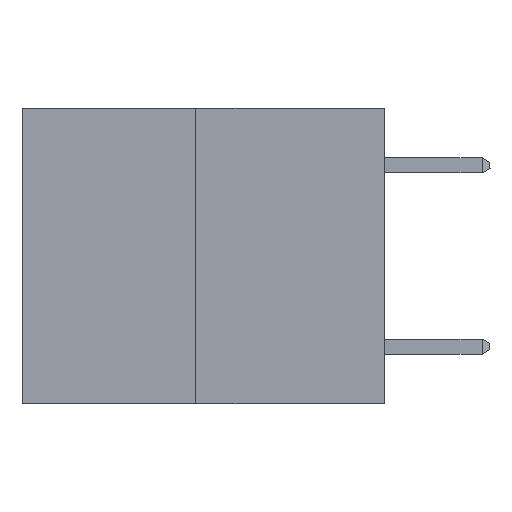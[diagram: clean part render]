
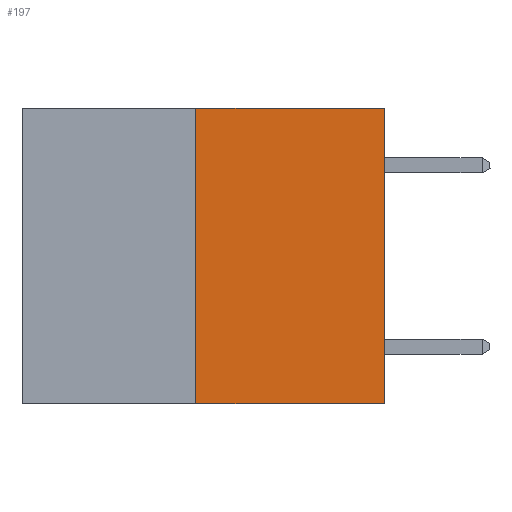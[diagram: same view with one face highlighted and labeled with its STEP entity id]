
A CAD part, left-side view. The second image highlights one B-rep face of the part: STEP entity #197.
In plain terms, the highlighted planar face has unit normal (-1, 0, 0).
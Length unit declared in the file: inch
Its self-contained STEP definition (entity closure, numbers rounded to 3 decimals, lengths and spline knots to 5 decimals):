
#197 = ADVANCED_FACE ( 'NONE', ( #6994 ), #12703, .F. ) ;
#657 = EDGE_CURVE ( 'NONE', #4104, #23526, #6106, .T. ) ;
#1776 = ORIENTED_EDGE ( 'NONE', *, *, #21878, .F. ) ;
#2484 = CARTESIAN_POINT ( 'NONE',  ( 0., 0., 0. ) ) ;
#3406 = DIRECTION ( 'NONE',  ( 0., -1., 0. ) ) ;
#3558 = VECTOR ( 'NONE', #4416, 39.37008 ) ;
#4104 = VERTEX_POINT ( 'NONE', #7059 ) ;
#4416 = DIRECTION ( 'NONE',  ( 0., -1., 0. ) ) ;
#5188 = VERTEX_POINT ( 'NONE', #6905 ) ;
#5438 = DIRECTION ( 'NONE',  ( 0., 0., 1. ) ) ;
#6106 = LINE ( 'NONE', #8871, #13394 ) ;
#6528 = AXIS2_PLACEMENT_3D ( 'NONE', #10986, #14589, #16468 ) ;
#6905 = CARTESIAN_POINT ( 'NONE',  ( 0., 0.312, 0. ) ) ;
#6994 = FACE_OUTER_BOUND ( 'NONE', #17328, .T. ) ;
#7059 = CARTESIAN_POINT ( 'NONE',  ( 0., 0.312, -0.49 ) ) ;
#7133 = ORIENTED_EDGE ( 'NONE', *, *, #657, .T. ) ;
#8530 = LINE ( 'NONE', #19288, #3558 ) ;
#8871 = CARTESIAN_POINT ( 'NONE',  ( 0., 0.6, -0.49 ) ) ;
#10242 = LINE ( 'NONE', #16699, #11083 ) ;
#10986 = CARTESIAN_POINT ( 'NONE',  ( 0., 0.6, 0. ) ) ;
#11083 = VECTOR ( 'NONE', #21775, 39.37008 ) ;
#12304 = VERTEX_POINT ( 'NONE', #2484 ) ;
#12703 = PLANE ( 'NONE',  #6528 ) ;
#13394 = VECTOR ( 'NONE', #3406, 39.37008 ) ;
#13621 = LINE ( 'NONE', #20406, #19517 ) ;
#14589 = DIRECTION ( 'NONE',  ( 1., 0., 0. ) ) ;
#16468 = DIRECTION ( 'NONE',  ( 0., 0., -1. ) ) ;
#16699 = CARTESIAN_POINT ( 'NONE',  ( 0., 0.312, -0.49 ) ) ;
#16796 = ORIENTED_EDGE ( 'NONE', *, *, #17579, .T. ) ;
#17328 = EDGE_LOOP ( 'NONE', ( #18672, #7133, #16796, #1776 ) ) ;
#17579 = EDGE_CURVE ( 'NONE', #23526, #12304, #13621, .T. ) ;
#18672 = ORIENTED_EDGE ( 'NONE', *, *, #22275, .F. ) ;
#19059 = CARTESIAN_POINT ( 'NONE',  ( 0., 0., -0.49 ) ) ;
#19288 = CARTESIAN_POINT ( 'NONE',  ( 0., 0.6, 0. ) ) ;
#19517 = VECTOR ( 'NONE', #5438, 39.37008 ) ;
#20406 = CARTESIAN_POINT ( 'NONE',  ( 0., 0., 0. ) ) ;
#21775 = DIRECTION ( 'NONE',  ( 0., 0., 1. ) ) ;
#21878 = EDGE_CURVE ( 'NONE', #5188, #12304, #8530, .T. ) ;
#22275 = EDGE_CURVE ( 'NONE', #4104, #5188, #10242, .T. ) ;
#23526 = VERTEX_POINT ( 'NONE', #19059 ) ;
